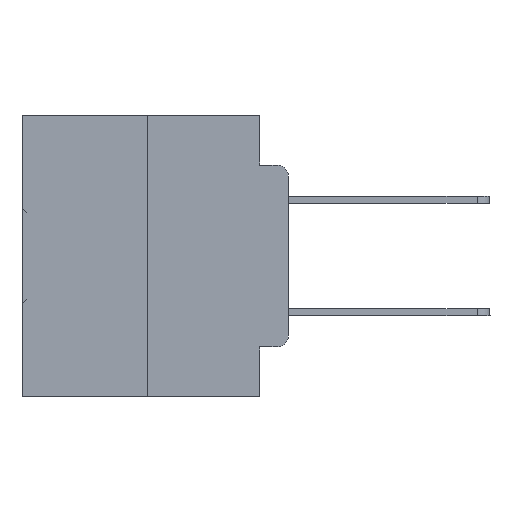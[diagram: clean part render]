
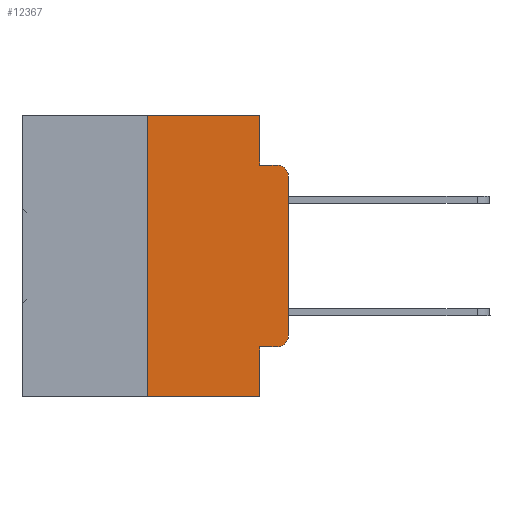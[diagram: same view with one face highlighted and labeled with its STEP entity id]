
A CAD part, left-side view. The second image highlights one B-rep face of the part: STEP entity #12367.
In plain terms, the highlighted planar face has unit normal (-1, 0, 0).
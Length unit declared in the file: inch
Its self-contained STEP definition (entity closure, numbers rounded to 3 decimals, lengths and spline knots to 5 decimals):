
#95 = CARTESIAN_POINT ( 'NONE',  ( 0., 0.051, -0.0885 ) ) ;
#625 = CARTESIAN_POINT ( 'NONE',  ( 0., 0.473, -0.5 ) ) ;
#1267 = DIRECTION ( 'NONE',  ( 1., 0., 0. ) ) ;
#1328 = VERTEX_POINT ( 'NONE', #35763 ) ;
#1707 = DIRECTION ( 'NONE',  ( 0., 0., -1. ) ) ;
#1881 = EDGE_CURVE ( 'NONE', #26305, #23864, #26089, .T. ) ;
#2225 = EDGE_LOOP ( 'NONE', ( #31719, #16030, #25414, #18014, #11192, #17589, #16125, #19724, #34293, #21933 ) ) ;
#2426 = CARTESIAN_POINT ( 'NONE',  ( 0., 0.02, -0.0885 ) ) ;
#2582 = LINE ( 'NONE', #6103, #34075 ) ;
#3359 = EDGE_CURVE ( 'NONE', #4607, #32697, #22028, .T. ) ;
#4026 = LINE ( 'NONE', #5199, #20348 ) ;
#4607 = VERTEX_POINT ( 'NONE', #12795 ) ;
#4994 = CIRCLE ( 'NONE', #16382, 0.02 ) ;
#5079 = EDGE_CURVE ( 'NONE', #10682, #1328, #12887, .T. ) ;
#5199 = CARTESIAN_POINT ( 'NONE',  ( 0., 0., 0. ) ) ;
#5495 = EDGE_CURVE ( 'NONE', #10682, #17592, #18728, .T. ) ;
#6103 = CARTESIAN_POINT ( 'NONE',  ( 0., 0.051, -0.0885 ) ) ;
#6523 = DIRECTION ( 'NONE',  ( 0., -1., 0. ) ) ;
#7768 = LINE ( 'NONE', #33569, #12096 ) ;
#8787 = VECTOR ( 'NONE', #1707, 39.37008 ) ;
#8882 = CARTESIAN_POINT ( 'NONE',  ( 0., 0.02, -0.4115 ) ) ;
#9215 = CARTESIAN_POINT ( 'NONE',  ( 0., 0.25, 0. ) ) ;
#9680 = DIRECTION ( 'NONE',  ( 0., 0., -1. ) ) ;
#10403 = VERTEX_POINT ( 'NONE', #33564 ) ;
#10682 = VERTEX_POINT ( 'NONE', #16744 ) ;
#11192 = ORIENTED_EDGE ( 'NONE', *, *, #32710, .F. ) ;
#11763 = DIRECTION ( 'NONE',  ( 0., -1., 0. ) ) ;
#12096 = VECTOR ( 'NONE', #25264, 39.37008 ) ;
#12299 = CARTESIAN_POINT ( 'NONE',  ( 0., 0.051, -0.5 ) ) ;
#12367 = ADVANCED_FACE ( 'NONE', ( #14080 ), #31646, .F. ) ;
#12795 = CARTESIAN_POINT ( 'NONE',  ( 0., 0.051, 0. ) ) ;
#12887 = LINE ( 'NONE', #9215, #27954 ) ;
#13107 = AXIS2_PLACEMENT_3D ( 'NONE', #25596, #24815, #29916 ) ;
#13485 = DIRECTION ( 'NONE',  ( 0., 0., -1. ) ) ;
#14080 = FACE_OUTER_BOUND ( 'NONE', #2225, .T. ) ;
#14208 = EDGE_CURVE ( 'NONE', #10403, #26305, #4026, .T. ) ;
#14666 = VECTOR ( 'NONE', #26525, 39.37008 ) ;
#14982 = CARTESIAN_POINT ( 'NONE',  ( 0., 0., -0.1085 ) ) ;
#15479 = CARTESIAN_POINT ( 'NONE',  ( 0., 0.051, 0. ) ) ;
#15487 = CARTESIAN_POINT ( 'NONE',  ( 0., 0.051, 0. ) ) ;
#15652 = CARTESIAN_POINT ( 'NONE',  ( 0., 0.051, -0.4115 ) ) ;
#16030 = ORIENTED_EDGE ( 'NONE', *, *, #1881, .T. ) ;
#16125 = ORIENTED_EDGE ( 'NONE', *, *, #5495, .T. ) ;
#16382 = AXIS2_PLACEMENT_3D ( 'NONE', #32577, #29661, #13485 ) ;
#16744 = CARTESIAN_POINT ( 'NONE',  ( 0., 0.25, -0.5 ) ) ;
#16970 = LINE ( 'NONE', #15479, #8787 ) ;
#17026 = CARTESIAN_POINT ( 'NONE',  ( 0., 0.051, -0.4115 ) ) ;
#17589 = ORIENTED_EDGE ( 'NONE', *, *, #5079, .F. ) ;
#17592 = VERTEX_POINT ( 'NONE', #12299 ) ;
#17776 = EDGE_CURVE ( 'NONE', #19689, #10403, #4994, .T. ) ;
#17870 = DIRECTION ( 'NONE',  ( 0., 0., 1. ) ) ;
#18014 = ORIENTED_EDGE ( 'NONE', *, *, #3359, .F. ) ;
#18728 = LINE ( 'NONE', #625, #23443 ) ;
#19689 = VERTEX_POINT ( 'NONE', #8882 ) ;
#19724 = ORIENTED_EDGE ( 'NONE', *, *, #34593, .F. ) ;
#20348 = VECTOR ( 'NONE', #26892, 39.37008 ) ;
#20617 = AXIS2_PLACEMENT_3D ( 'NONE', #34384, #1267, #9680 ) ;
#21233 = VECTOR ( 'NONE', #11763, 39.37008 ) ;
#21933 = ORIENTED_EDGE ( 'NONE', *, *, #17776, .T. ) ;
#22028 = LINE ( 'NONE', #15487, #14666 ) ;
#23050 = DIRECTION ( 'NONE',  ( 0., -1., 0. ) ) ;
#23435 = EDGE_CURVE ( 'NONE', #32697, #23864, #2582, .T. ) ;
#23443 = VECTOR ( 'NONE', #6523, 39.37008 ) ;
#23864 = VERTEX_POINT ( 'NONE', #2426 ) ;
#24269 = LINE ( 'NONE', #17026, #21233 ) ;
#24815 = DIRECTION ( 'NONE',  ( -1., 0., 0. ) ) ;
#25205 = VERTEX_POINT ( 'NONE', #15652 ) ;
#25264 = DIRECTION ( 'NONE',  ( 0., -1., 0. ) ) ;
#25414 = ORIENTED_EDGE ( 'NONE', *, *, #23435, .F. ) ;
#25596 = CARTESIAN_POINT ( 'NONE',  ( 0., 0.02, -0.1085 ) ) ;
#26089 = CIRCLE ( 'NONE', #13107, 0.02 ) ;
#26305 = VERTEX_POINT ( 'NONE', #14982 ) ;
#26525 = DIRECTION ( 'NONE',  ( 0., 0., -1. ) ) ;
#26892 = DIRECTION ( 'NONE',  ( 0., 0., 1. ) ) ;
#27954 = VECTOR ( 'NONE', #17870, 39.37008 ) ;
#29661 = DIRECTION ( 'NONE',  ( -1., 0., 0. ) ) ;
#29916 = DIRECTION ( 'NONE',  ( 0., 0., -1. ) ) ;
#31315 = EDGE_CURVE ( 'NONE', #25205, #19689, #24269, .T. ) ;
#31646 = PLANE ( 'NONE',  #20617 ) ;
#31719 = ORIENTED_EDGE ( 'NONE', *, *, #14208, .T. ) ;
#32577 = CARTESIAN_POINT ( 'NONE',  ( 0., 0.02, -0.3915 ) ) ;
#32697 = VERTEX_POINT ( 'NONE', #95 ) ;
#32710 = EDGE_CURVE ( 'NONE', #1328, #4607, #7768, .T. ) ;
#33564 = CARTESIAN_POINT ( 'NONE',  ( 0., 0., -0.3915 ) ) ;
#33569 = CARTESIAN_POINT ( 'NONE',  ( 0., 0.473, 0. ) ) ;
#34075 = VECTOR ( 'NONE', #23050, 39.37008 ) ;
#34293 = ORIENTED_EDGE ( 'NONE', *, *, #31315, .T. ) ;
#34384 = CARTESIAN_POINT ( 'NONE',  ( 0., 0.473, 0. ) ) ;
#34593 = EDGE_CURVE ( 'NONE', #25205, #17592, #16970, .T. ) ;
#35763 = CARTESIAN_POINT ( 'NONE',  ( 0., 0.25, 0. ) ) ;
